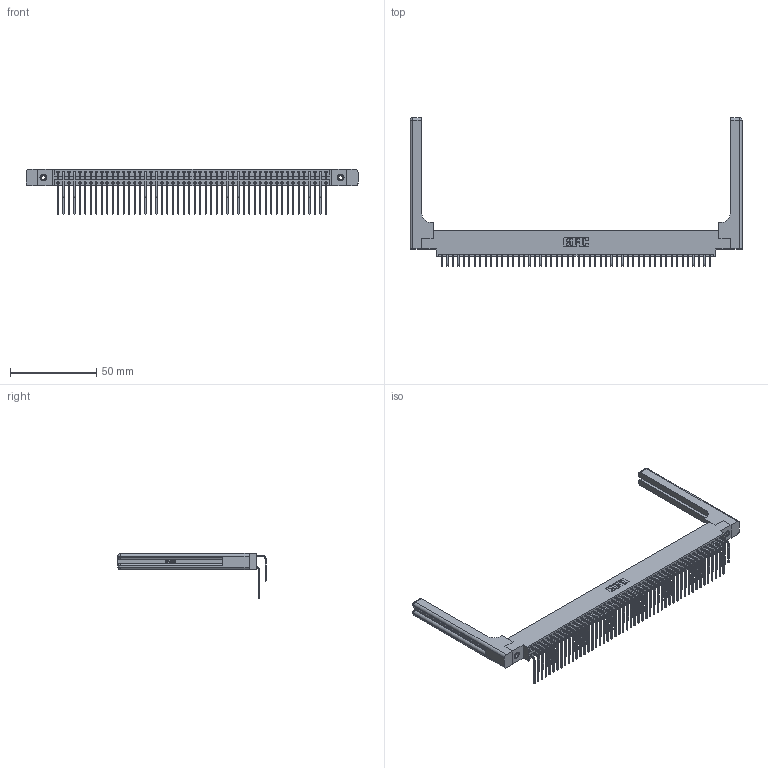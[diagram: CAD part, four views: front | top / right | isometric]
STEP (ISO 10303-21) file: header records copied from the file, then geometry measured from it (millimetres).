
FILE_DESCRIPTION (( 'STEP AP203' ), '1' );
FILE_NAME ('396-100-559-858.STEP', '2019-11-03T16:16:55', ( '' ), ( '' ), 'SwSTEP 2.0', 'SolidWorks 2016', '' );
FILE_SCHEMA (( 'CONFIG_CONTROL_DESIGN' ));
Length unit declared in the file: inch
Products named in the file (6): 346 Part_0.170 Offset - 0.156 Dia-TH; 345-292-001_558 559 Tail - 1; 345-250-001_345-250-001-102; 345-292-001_559 Tail - 2; 396-100-559-858; 346-220-058_345-220-058
Assembly tree (105 placements, depth 2):
  396-100-559-858
    346 Part_0.170 Offset - 0.156 Dia-TH
    345-292-001_558 559 Tail - 1  x50
    345-292-001_559 Tail - 2  x50
    345-250-001_345-250-001-102  x2
    346-220-058_345-220-058  x2
Bounding box: 192.81 x 86.17 x 26.16 mm (x, y, z)
Volume: 26780.1 mm3; surface area: 34555.4 mm2
Topology: 105 solids, 105 shells, 5782 faces, 17107 edges, 11250 vertices
Faces by surface type: plane 3928, cylinder 1794, bspline 36, cone 12, sphere 8, torus 4
Entity records: 38652 total; most frequent: CARTESIAN_POINT 7420, ORIENTED_EDGE 6100, DIRECTION 5494, EDGE_CURVE 3050, LINE 2586, VECTOR 2586, VERTEX_POINT 2022, AXIS2_PLACEMENT_3D 1454
